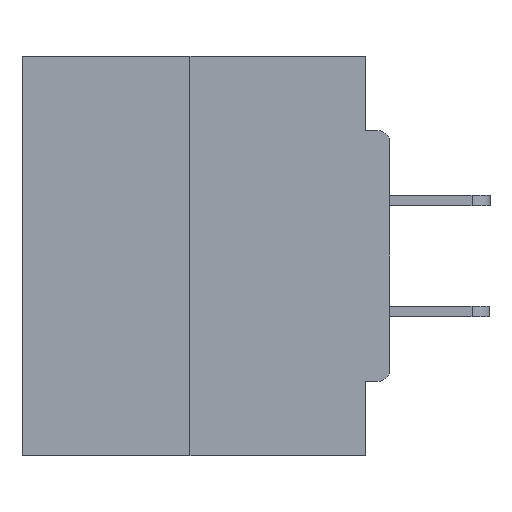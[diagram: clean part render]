
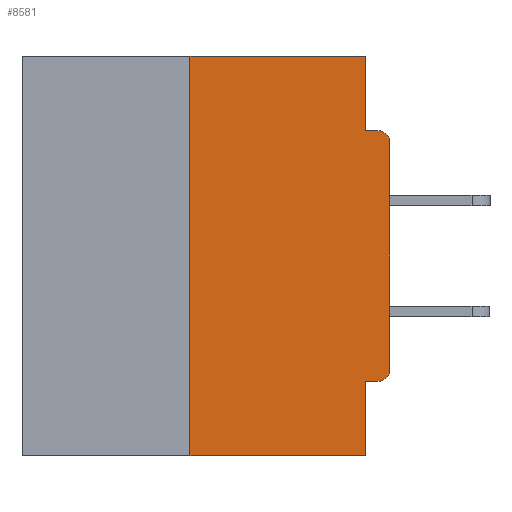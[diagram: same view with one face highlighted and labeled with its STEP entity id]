
A CAD part, left-side view. The second image highlights one B-rep face of the part: STEP entity #8581.
In plain terms, the highlighted planar face has unit normal (-1, 0, 0).
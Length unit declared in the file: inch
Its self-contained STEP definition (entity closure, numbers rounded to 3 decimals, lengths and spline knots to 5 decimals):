
#121 = CARTESIAN_POINT ( 'NONE',  ( 0., 0.031, 0. ) ) ;
#914 = CARTESIAN_POINT ( 'NONE',  ( 0., 0., -0.3915 ) ) ;
#1415 = LINE ( 'NONE', #17462, #10395 ) ;
#1984 = DIRECTION ( 'NONE',  ( 0., 1., 0. ) ) ;
#2155 = LINE ( 'NONE', #4870, #3395 ) ;
#2927 = CARTESIAN_POINT ( 'NONE',  ( 0., 0.015, -0.4065 ) ) ;
#3099 = VECTOR ( 'NONE', #25482, 39.37008 ) ;
#3163 = ORIENTED_EDGE ( 'NONE', *, *, #11265, .F. ) ;
#3395 = VECTOR ( 'NONE', #15059, 39.37008 ) ;
#4155 = EDGE_CURVE ( 'NONE', #20179, #15447, #33753, .T. ) ;
#4870 = CARTESIAN_POINT ( 'NONE',  ( 0., 0., 0. ) ) ;
#5063 = CARTESIAN_POINT ( 'NONE',  ( 0., 0.015, -0.1085 ) ) ;
#5570 = ORIENTED_EDGE ( 'NONE', *, *, #30311, .F. ) ;
#5610 = ORIENTED_EDGE ( 'NONE', *, *, #4155, .F. ) ;
#5964 = CIRCLE ( 'NONE', #15289, 0.015 ) ;
#6387 = CARTESIAN_POINT ( 'NONE',  ( 0., 0.031, -0.0935 ) ) ;
#6504 = EDGE_LOOP ( 'NONE', ( #27328, #11985, #28011, #5570, #3163, #25764, #31300, #16678, #12298, #5610 ) ) ;
#7431 = CARTESIAN_POINT ( 'NONE',  ( 0., 0.46, -0.5 ) ) ;
#7493 = DIRECTION ( 'NONE',  ( 0., 0., -1. ) ) ;
#7685 = EDGE_CURVE ( 'NONE', #9460, #8222, #5964, .T. ) ;
#8222 = VERTEX_POINT ( 'NONE', #26704 ) ;
#8581 = ADVANCED_FACE ( 'NONE', ( #23055 ), #33349, .F. ) ;
#8884 = VECTOR ( 'NONE', #1984, 39.37008 ) ;
#9460 = VERTEX_POINT ( 'NONE', #27648 ) ;
#10093 = VECTOR ( 'NONE', #10695, 39.37008 ) ;
#10117 = VERTEX_POINT ( 'NONE', #13279 ) ;
#10395 = VECTOR ( 'NONE', #25956, 39.37008 ) ;
#10695 = DIRECTION ( 'NONE',  ( 0., -1., 0. ) ) ;
#10789 = CARTESIAN_POINT ( 'NONE',  ( 0., 0.25, -0.5 ) ) ;
#11265 = EDGE_CURVE ( 'NONE', #19724, #31288, #33126, .T. ) ;
#11447 = DIRECTION ( 'NONE',  ( -1., 0., 0. ) ) ;
#11589 = LINE ( 'NONE', #14220, #17736 ) ;
#11985 = ORIENTED_EDGE ( 'NONE', *, *, #18788, .F. ) ;
#12298 = ORIENTED_EDGE ( 'NONE', *, *, #22155, .F. ) ;
#12406 = DIRECTION ( 'NONE',  ( 0., 0., -1. ) ) ;
#13051 = DIRECTION ( 'NONE',  ( 0., 0., -1. ) ) ;
#13279 = CARTESIAN_POINT ( 'NONE',  ( 0., 0.031, -0.5 ) ) ;
#14220 = CARTESIAN_POINT ( 'NONE',  ( 0., 0.25, 0. ) ) ;
#15059 = DIRECTION ( 'NONE',  ( 0., 0., 1. ) ) ;
#15289 = AXIS2_PLACEMENT_3D ( 'NONE', #5063, #15716, #13051 ) ;
#15447 = VERTEX_POINT ( 'NONE', #6387 ) ;
#15716 = DIRECTION ( 'NONE',  ( -1., 0., 0. ) ) ;
#15903 = EDGE_CURVE ( 'NONE', #20288, #10117, #32737, .T. ) ;
#16678 = ORIENTED_EDGE ( 'NONE', *, *, #7685, .T. ) ;
#17462 = CARTESIAN_POINT ( 'NONE',  ( 0., 0.46, 0. ) ) ;
#17736 = VECTOR ( 'NONE', #19301, 39.37008 ) ;
#17884 = CARTESIAN_POINT ( 'NONE',  ( 0., 0., -0.0935 ) ) ;
#18496 = EDGE_CURVE ( 'NONE', #21998, #9460, #2155, .T. ) ;
#18788 = EDGE_CURVE ( 'NONE', #20288, #33131, #11589, .T. ) ;
#19301 = DIRECTION ( 'NONE',  ( 0., 0., 1. ) ) ;
#19724 = VERTEX_POINT ( 'NONE', #2927 ) ;
#20179 = VERTEX_POINT ( 'NONE', #121 ) ;
#20288 = VERTEX_POINT ( 'NONE', #10789 ) ;
#20431 = DIRECTION ( 'NONE',  ( 0., -1., 0. ) ) ;
#21401 = VECTOR ( 'NONE', #20431, 39.37008 ) ;
#21998 = VERTEX_POINT ( 'NONE', #914 ) ;
#22155 = EDGE_CURVE ( 'NONE', #15447, #8222, #24668, .T. ) ;
#22168 = AXIS2_PLACEMENT_3D ( 'NONE', #22775, #23003, #12406 ) ;
#22775 = CARTESIAN_POINT ( 'NONE',  ( 0., 0.46, 0. ) ) ;
#22987 = CARTESIAN_POINT ( 'NONE',  ( 0., 0.031, 0. ) ) ;
#23003 = DIRECTION ( 'NONE',  ( 1., 0., 0. ) ) ;
#23055 = FACE_OUTER_BOUND ( 'NONE', #6504, .T. ) ;
#24376 = AXIS2_PLACEMENT_3D ( 'NONE', #29594, #11447, #27112 ) ;
#24668 = LINE ( 'NONE', #17884, #21401 ) ;
#25482 = DIRECTION ( 'NONE',  ( 0., 0., -1. ) ) ;
#25764 = ORIENTED_EDGE ( 'NONE', *, *, #27843, .T. ) ;
#25956 = DIRECTION ( 'NONE',  ( 0., -1., 0. ) ) ;
#26704 = CARTESIAN_POINT ( 'NONE',  ( 0., 0.015, -0.0935 ) ) ;
#26765 = VECTOR ( 'NONE', #7493, 39.37008 ) ;
#27112 = DIRECTION ( 'NONE',  ( 0., 0., -1. ) ) ;
#27328 = ORIENTED_EDGE ( 'NONE', *, *, #30764, .F. ) ;
#27648 = CARTESIAN_POINT ( 'NONE',  ( 0., 0., -0.1085 ) ) ;
#27787 = LINE ( 'NONE', #30519, #3099 ) ;
#27795 = CARTESIAN_POINT ( 'NONE',  ( 0., 0.031, -0.4065 ) ) ;
#27843 = EDGE_CURVE ( 'NONE', #19724, #21998, #33748, .T. ) ;
#28011 = ORIENTED_EDGE ( 'NONE', *, *, #15903, .T. ) ;
#29139 = CARTESIAN_POINT ( 'NONE',  ( 0., 0.25, 0. ) ) ;
#29594 = CARTESIAN_POINT ( 'NONE',  ( 0., 0.015, -0.3915 ) ) ;
#30311 = EDGE_CURVE ( 'NONE', #31288, #10117, #27787, .T. ) ;
#30519 = CARTESIAN_POINT ( 'NONE',  ( 0., 0.031, -0.5 ) ) ;
#30764 = EDGE_CURVE ( 'NONE', #33131, #20179, #1415, .T. ) ;
#31288 = VERTEX_POINT ( 'NONE', #27795 ) ;
#31300 = ORIENTED_EDGE ( 'NONE', *, *, #18496, .T. ) ;
#32737 = LINE ( 'NONE', #7431, #10093 ) ;
#33126 = LINE ( 'NONE', #33453, #8884 ) ;
#33131 = VERTEX_POINT ( 'NONE', #29139 ) ;
#33349 = PLANE ( 'NONE',  #22168 ) ;
#33453 = CARTESIAN_POINT ( 'NONE',  ( 0., 0., -0.4065 ) ) ;
#33748 = CIRCLE ( 'NONE', #24376, 0.015 ) ;
#33753 = LINE ( 'NONE', #22987, #26765 ) ;
